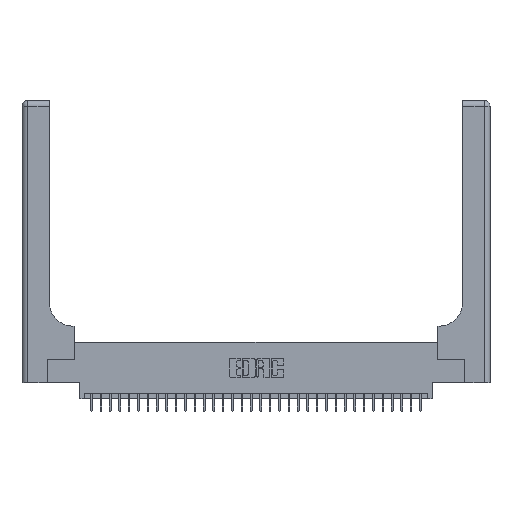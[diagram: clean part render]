
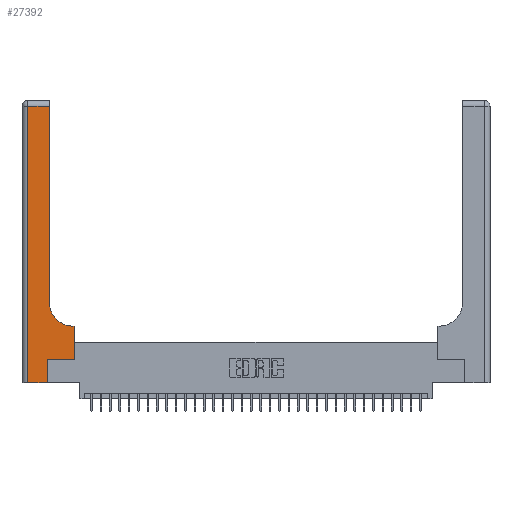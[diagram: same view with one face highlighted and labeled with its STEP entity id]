
A CAD part, top view. The second image highlights one B-rep face of the part: STEP entity #27392.
In plain terms, the highlighted planar face has unit normal (0, 0, 1).
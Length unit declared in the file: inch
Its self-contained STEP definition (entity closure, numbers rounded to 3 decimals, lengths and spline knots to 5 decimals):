
#1158 = CARTESIAN_POINT ( 'NONE',  ( 0.2915, 0.85, 0.37 ) ) ;
#1289 = LINE ( 'NONE', #1813, #2177 ) ;
#1345 = ORIENTED_EDGE ( 'NONE', *, *, #20361, .T. ) ;
#1813 = CARTESIAN_POINT ( 'NONE',  ( 0.5585, 0.25, 0.37 ) ) ;
#2177 = VECTOR ( 'NONE', #17525, 39.37008 ) ;
#2215 = EDGE_CURVE ( 'NONE', #6278, #20548, #33767, .T. ) ;
#2791 = LINE ( 'NONE', #6131, #9442 ) ;
#3415 = AXIS2_PLACEMENT_3D ( 'NONE', #17546, #12296, #14742 ) ;
#3792 = CARTESIAN_POINT ( 'NONE',  ( 0.269, 0., 0.37 ) ) ;
#4534 = DIRECTION ( 'NONE',  ( -1., 0., 0. ) ) ;
#4665 = EDGE_LOOP ( 'NONE', ( #21928, #10244, #1345, #5395, #26307, #20151, #9733, #5551, #8875 ) ) ;
#5395 = ORIENTED_EDGE ( 'NONE', *, *, #2215, .T. ) ;
#5551 = ORIENTED_EDGE ( 'NONE', *, *, #6595, .T. ) ;
#5883 = VERTEX_POINT ( 'NONE', #16312 ) ;
#5961 = EDGE_CURVE ( 'NONE', #6727, #16879, #1289, .T. ) ;
#6131 = CARTESIAN_POINT ( 'NONE',  ( 0.2915, 0.6, 0.37 ) ) ;
#6203 = VECTOR ( 'NONE', #33991, 39.37008 ) ;
#6278 = VERTEX_POINT ( 'NONE', #27126 ) ;
#6595 = EDGE_CURVE ( 'NONE', #16879, #27876, #2791, .T. ) ;
#6727 = VERTEX_POINT ( 'NONE', #33141 ) ;
#7993 = LINE ( 'NONE', #10254, #6203 ) ;
#8875 = ORIENTED_EDGE ( 'NONE', *, *, #29418, .T. ) ;
#8970 = DIRECTION ( 'NONE',  ( 0., 1., 0. ) ) ;
#9442 = VECTOR ( 'NONE', #29347, 39.37008 ) ;
#9733 = ORIENTED_EDGE ( 'NONE', *, *, #5961, .T. ) ;
#9940 = CARTESIAN_POINT ( 'NONE',  ( 0., 3., 0.37 ) ) ;
#10244 = ORIENTED_EDGE ( 'NONE', *, *, #30336, .T. ) ;
#10254 = CARTESIAN_POINT ( 'NONE',  ( 0., 2.94, 0.37 ) ) ;
#10273 = FACE_OUTER_BOUND ( 'NONE', #4665, .T. ) ;
#10389 = LINE ( 'NONE', #20226, #21302 ) ;
#10748 = CARTESIAN_POINT ( 'NONE',  ( 0.5415, 0.6, 0.37 ) ) ;
#12296 = DIRECTION ( 'NONE',  ( 0., 0., -1. ) ) ;
#13202 = EDGE_CURVE ( 'NONE', #20548, #21056, #20187, .T. ) ;
#13293 = VERTEX_POINT ( 'NONE', #1158 ) ;
#14742 = DIRECTION ( 'NONE',  ( 1., 0., 0. ) ) ;
#16165 = EDGE_CURVE ( 'NONE', #13293, #16468, #29571, .T. ) ;
#16312 = CARTESIAN_POINT ( 'NONE',  ( 0.06, 2.94, 0.37 ) ) ;
#16468 = VERTEX_POINT ( 'NONE', #18556 ) ;
#16879 = VERTEX_POINT ( 'NONE', #27871 ) ;
#17525 = DIRECTION ( 'NONE',  ( 0., 1., 0. ) ) ;
#17546 = CARTESIAN_POINT ( 'NONE',  ( 0.5415, 0.85, 0.37 ) ) ;
#17636 = AXIS2_PLACEMENT_3D ( 'NONE', #9940, #28455, #4534 ) ;
#17855 = CARTESIAN_POINT ( 'NONE',  ( 0.269, 0.25, 0.37 ) ) ;
#18475 = CIRCLE ( 'NONE', #3415, 0.25 ) ;
#18556 = CARTESIAN_POINT ( 'NONE',  ( 0.2915, 2.94, 0.37 ) ) ;
#19267 = CARTESIAN_POINT ( 'NONE',  ( 0.2915, 3., 0.37 ) ) ;
#20047 = VECTOR ( 'NONE', #8970, 39.37008 ) ;
#20151 = ORIENTED_EDGE ( 'NONE', *, *, #29889, .T. ) ;
#20187 = LINE ( 'NONE', #3792, #27091 ) ;
#20226 = CARTESIAN_POINT ( 'NONE',  ( 0.06, 3., 0.37 ) ) ;
#20361 = EDGE_CURVE ( 'NONE', #5883, #6278, #10389, .T. ) ;
#20548 = VERTEX_POINT ( 'NONE', #25571 ) ;
#21054 = DIRECTION ( 'NONE',  ( 0., -1., 0. ) ) ;
#21056 = VERTEX_POINT ( 'NONE', #27970 ) ;
#21302 = VECTOR ( 'NONE', #21054, 39.37008 ) ;
#21928 = ORIENTED_EDGE ( 'NONE', *, *, #16165, .T. ) ;
#25230 = VECTOR ( 'NONE', #25384, 39.37008 ) ;
#25384 = DIRECTION ( 'NONE',  ( 1., 0., 0. ) ) ;
#25571 = CARTESIAN_POINT ( 'NONE',  ( 0.269, 0., 0.37 ) ) ;
#25767 = DIRECTION ( 'NONE',  ( 1., 0., 0. ) ) ;
#26307 = ORIENTED_EDGE ( 'NONE', *, *, #13202, .T. ) ;
#27091 = VECTOR ( 'NONE', #27886, 39.37008 ) ;
#27126 = CARTESIAN_POINT ( 'NONE',  ( 0.06, 0., 0.37 ) ) ;
#27392 = ADVANCED_FACE ( 'NONE', ( #10273 ), #33843, .F. ) ;
#27871 = CARTESIAN_POINT ( 'NONE',  ( 0.5585, 0.6, 0.37 ) ) ;
#27876 = VERTEX_POINT ( 'NONE', #10748 ) ;
#27886 = DIRECTION ( 'NONE',  ( 0., 1., 0. ) ) ;
#27970 = CARTESIAN_POINT ( 'NONE',  ( 0.269, 0.25, 0.37 ) ) ;
#28195 = CARTESIAN_POINT ( 'NONE',  ( 0., 0., 0.37 ) ) ;
#28455 = DIRECTION ( 'NONE',  ( 0., 0., -1. ) ) ;
#29347 = DIRECTION ( 'NONE',  ( -1., 0., 0. ) ) ;
#29418 = EDGE_CURVE ( 'NONE', #27876, #13293, #18475, .T. ) ;
#29571 = LINE ( 'NONE', #19267, #20047 ) ;
#29889 = EDGE_CURVE ( 'NONE', #21056, #6727, #30606, .T. ) ;
#30336 = EDGE_CURVE ( 'NONE', #16468, #5883, #7993, .T. ) ;
#30606 = LINE ( 'NONE', #17855, #25230 ) ;
#32656 = VECTOR ( 'NONE', #25767, 39.37008 ) ;
#33141 = CARTESIAN_POINT ( 'NONE',  ( 0.5585, 0.25, 0.37 ) ) ;
#33767 = LINE ( 'NONE', #28195, #32656 ) ;
#33843 = PLANE ( 'NONE',  #17636 ) ;
#33991 = DIRECTION ( 'NONE',  ( -1., 0., 0. ) ) ;
